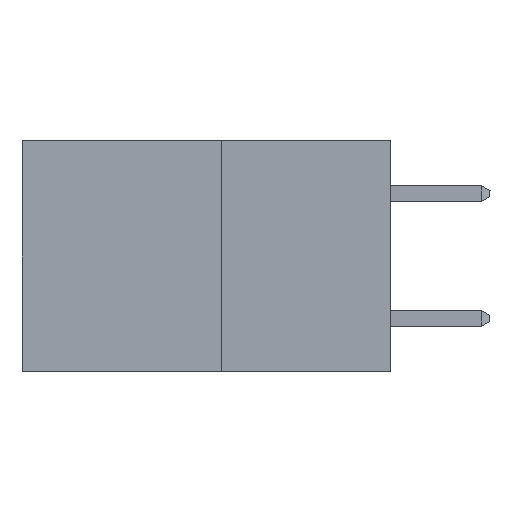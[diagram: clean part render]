
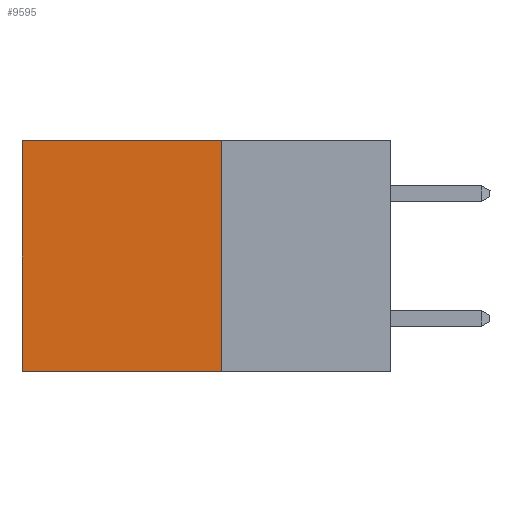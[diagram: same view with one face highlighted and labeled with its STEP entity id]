
A CAD part, left-side view. The second image highlights one B-rep face of the part: STEP entity #9595.
In plain terms, the highlighted planar face has unit normal (-1, 0, 0).
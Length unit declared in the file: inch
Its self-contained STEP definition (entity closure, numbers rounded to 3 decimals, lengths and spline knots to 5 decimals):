
#98 = PLANE ( 'NONE',  #1440 ) ;
#855 = FACE_OUTER_BOUND ( 'NONE', #5948, .T. ) ;
#920 = DIRECTION ( 'NONE',  ( 0., 0., -1. ) ) ;
#1411 = CARTESIAN_POINT ( 'NONE',  ( 0.277, 0.27, -0.37 ) ) ;
#1440 = AXIS2_PLACEMENT_3D ( 'NONE', #9482, #2483, #920 ) ;
#1793 = CARTESIAN_POINT ( 'NONE',  ( 0.277, 0.59, -0.37 ) ) ;
#1903 = VECTOR ( 'NONE', #7968, 39.37008 ) ;
#2390 = EDGE_CURVE ( 'NONE', #4640, #8531, #5298, .T. ) ;
#2483 = DIRECTION ( 'NONE',  ( 1., 0., 0. ) ) ;
#2686 = CARTESIAN_POINT ( 'NONE',  ( 0.277, 0.59, -0.37 ) ) ;
#2710 = DIRECTION ( 'NONE',  ( 0., 0., -1. ) ) ;
#2763 = ORIENTED_EDGE ( 'NONE', *, *, #10052, .F. ) ;
#3026 = CARTESIAN_POINT ( 'NONE',  ( 0.277, 0.27, 0. ) ) ;
#3669 = VECTOR ( 'NONE', #2710, 39.37008 ) ;
#4178 = CARTESIAN_POINT ( 'NONE',  ( 0.277, 0.27, 0. ) ) ;
#4592 = VECTOR ( 'NONE', #8540, 39.37008 ) ;
#4640 = VERTEX_POINT ( 'NONE', #4178 ) ;
#4840 = LINE ( 'NONE', #10004, #4592 ) ;
#5298 = LINE ( 'NONE', #3026, #9371 ) ;
#5539 = EDGE_CURVE ( 'NONE', #8531, #8504, #5762, .T. ) ;
#5691 = ORIENTED_EDGE ( 'NONE', *, *, #5539, .T. ) ;
#5762 = LINE ( 'NONE', #2686, #3669 ) ;
#5938 = ORIENTED_EDGE ( 'NONE', *, *, #2390, .T. ) ;
#5948 = EDGE_LOOP ( 'NONE', ( #5691, #7722, #2763, #5938 ) ) ;
#5990 = EDGE_CURVE ( 'NONE', #10005, #8504, #9476, .T. ) ;
#7722 = ORIENTED_EDGE ( 'NONE', *, *, #5990, .F. ) ;
#7968 = DIRECTION ( 'NONE',  ( 0., 1., 0. ) ) ;
#8052 = CARTESIAN_POINT ( 'NONE',  ( 0.277, 0.27, -0.37 ) ) ;
#8117 = CARTESIAN_POINT ( 'NONE',  ( 0.277, 0.59, 0. ) ) ;
#8504 = VERTEX_POINT ( 'NONE', #1793 ) ;
#8531 = VERTEX_POINT ( 'NONE', #8117 ) ;
#8540 = DIRECTION ( 'NONE',  ( 0., 0., -1. ) ) ;
#9228 = DIRECTION ( 'NONE',  ( 0., 1., 0. ) ) ;
#9371 = VECTOR ( 'NONE', #9228, 39.37008 ) ;
#9476 = LINE ( 'NONE', #8052, #1903 ) ;
#9482 = CARTESIAN_POINT ( 'NONE',  ( 0.277, 0.27, -0.37 ) ) ;
#9595 = ADVANCED_FACE ( 'NONE', ( #855 ), #98, .F. ) ;
#10004 = CARTESIAN_POINT ( 'NONE',  ( 0.277, 0.27, -0.37 ) ) ;
#10005 = VERTEX_POINT ( 'NONE', #1411 ) ;
#10052 = EDGE_CURVE ( 'NONE', #4640, #10005, #4840, .T. ) ;
